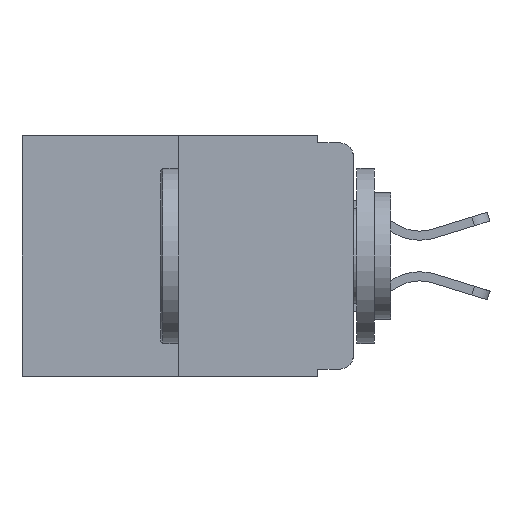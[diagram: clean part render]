
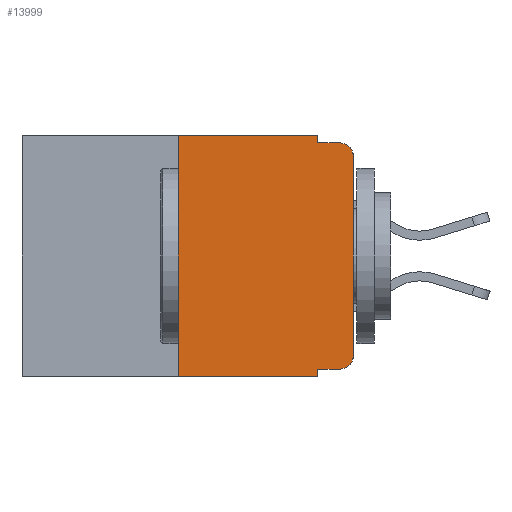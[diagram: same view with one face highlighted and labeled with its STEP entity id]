
A CAD part, left-side view. The second image highlights one B-rep face of the part: STEP entity #13999.
In plain terms, the highlighted planar face has unit normal (-1, 0, 0).
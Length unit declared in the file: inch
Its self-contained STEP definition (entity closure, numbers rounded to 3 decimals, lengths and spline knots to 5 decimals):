
#170 = CARTESIAN_POINT ( 'NONE',  ( 0., 0., -0.313 ) ) ;
#595 = EDGE_CURVE ( 'NONE', #14541, #14249, #4104, .T. ) ;
#627 = DIRECTION ( 'NONE',  ( 0., 0., -1. ) ) ;
#764 = VERTEX_POINT ( 'NONE', #4735 ) ;
#1036 = CARTESIAN_POINT ( 'NONE',  ( 0., 0.051, -0.343 ) ) ;
#1538 = CARTESIAN_POINT ( 'NONE',  ( 0., 0.051, -0.333 ) ) ;
#2058 = CARTESIAN_POINT ( 'NONE',  ( 0., 0.25, 0. ) ) ;
#2104 = CARTESIAN_POINT ( 'NONE',  ( 0., 0.051, 0. ) ) ;
#2351 = VECTOR ( 'NONE', #6844, 39.37008 ) ;
#2370 = VECTOR ( 'NONE', #8442, 39.37008 ) ;
#2421 = EDGE_CURVE ( 'NONE', #15066, #16653, #8781, .T. ) ;
#2644 = VECTOR ( 'NONE', #10840, 39.37008 ) ;
#3401 = CARTESIAN_POINT ( 'NONE',  ( 0., 0.051, 0. ) ) ;
#3480 = CARTESIAN_POINT ( 'NONE',  ( 0., 0.02, -0.313 ) ) ;
#3957 = AXIS2_PLACEMENT_3D ( 'NONE', #16062, #11904, #13245 ) ;
#4104 = CIRCLE ( 'NONE', #15993, 0.02 ) ;
#4123 = DIRECTION ( 'NONE',  ( 0., -1., 0. ) ) ;
#4286 = ORIENTED_EDGE ( 'NONE', *, *, #595, .T. ) ;
#4735 = CARTESIAN_POINT ( 'NONE',  ( 0., 0., -0.03 ) ) ;
#4946 = EDGE_CURVE ( 'NONE', #12644, #6397, #11073, .T. ) ;
#5188 = CARTESIAN_POINT ( 'NONE',  ( 0., 0.25, 0. ) ) ;
#5298 = ORIENTED_EDGE ( 'NONE', *, *, #17246, .F. ) ;
#5504 = CARTESIAN_POINT ( 'NONE',  ( 0., 0.051, 0. ) ) ;
#5694 = LINE ( 'NONE', #1538, #16495 ) ;
#5914 = FACE_OUTER_BOUND ( 'NONE', #6399, .T. ) ;
#6042 = ORIENTED_EDGE ( 'NONE', *, *, #4946, .F. ) ;
#6061 = DIRECTION ( 'NONE',  ( 0., -1., 0. ) ) ;
#6142 = CARTESIAN_POINT ( 'NONE',  ( 0., 0.02, -0.333 ) ) ;
#6217 = LINE ( 'NONE', #8803, #7564 ) ;
#6397 = VERTEX_POINT ( 'NONE', #13373 ) ;
#6399 = EDGE_LOOP ( 'NONE', ( #8392, #15746, #17805, #6042, #5298, #8787, #16891, #14525, #8882, #4286 ) ) ;
#6556 = EDGE_CURVE ( 'NONE', #7332, #14581, #12127, .T. ) ;
#6844 = DIRECTION ( 'NONE',  ( 0., 0., 1. ) ) ;
#6945 = CIRCLE ( 'NONE', #9717, 0.02 ) ;
#7332 = VERTEX_POINT ( 'NONE', #9834 ) ;
#7340 = LINE ( 'NONE', #10999, #2370 ) ;
#7564 = VECTOR ( 'NONE', #6061, 39.37008 ) ;
#7791 = VERTEX_POINT ( 'NONE', #17828 ) ;
#8173 = CARTESIAN_POINT ( 'NONE',  ( 0., 0.051, -0.01 ) ) ;
#8340 = DIRECTION ( 'NONE',  ( 0., -1., 0. ) ) ;
#8392 = ORIENTED_EDGE ( 'NONE', *, *, #17815, .T. ) ;
#8442 = DIRECTION ( 'NONE',  ( 0., -1., 0. ) ) ;
#8781 = LINE ( 'NONE', #5504, #13330 ) ;
#8787 = ORIENTED_EDGE ( 'NONE', *, *, #6556, .F. ) ;
#8803 = CARTESIAN_POINT ( 'NONE',  ( 0., 0.473, -0.343 ) ) ;
#8882 = ORIENTED_EDGE ( 'NONE', *, *, #14210, .T. ) ;
#9075 = VECTOR ( 'NONE', #8340, 39.37008 ) ;
#9501 = DIRECTION ( 'NONE',  ( 0., 0., -1. ) ) ;
#9717 = AXIS2_PLACEMENT_3D ( 'NONE', #17316, #16001, #14624 ) ;
#9834 = CARTESIAN_POINT ( 'NONE',  ( 0., 0.25, -0.343 ) ) ;
#10254 = DIRECTION ( 'NONE',  ( 0., 0., -1. ) ) ;
#10840 = DIRECTION ( 'NONE',  ( 0., 0., 1. ) ) ;
#10854 = CARTESIAN_POINT ( 'NONE',  ( 0., 0., 0. ) ) ;
#10999 = CARTESIAN_POINT ( 'NONE',  ( 0., 0.473, 0. ) ) ;
#11073 = LINE ( 'NONE', #3401, #13444 ) ;
#11733 = PLANE ( 'NONE',  #3957 ) ;
#11904 = DIRECTION ( 'NONE',  ( 1., 0., 0. ) ) ;
#12127 = LINE ( 'NONE', #5188, #2644 ) ;
#12268 = EDGE_CURVE ( 'NONE', #764, #7791, #6945, .T. ) ;
#12644 = VERTEX_POINT ( 'NONE', #2104 ) ;
#12970 = CARTESIAN_POINT ( 'NONE',  ( 0., 0.051, -0.333 ) ) ;
#13245 = DIRECTION ( 'NONE',  ( 0., 0., -1. ) ) ;
#13330 = VECTOR ( 'NONE', #9501, 39.37008 ) ;
#13373 = CARTESIAN_POINT ( 'NONE',  ( 0., 0.051, -0.01 ) ) ;
#13376 = LINE ( 'NONE', #10854, #2351 ) ;
#13444 = VECTOR ( 'NONE', #627, 39.37008 ) ;
#13999 = ADVANCED_FACE ( 'NONE', ( #5914 ), #11733, .F. ) ;
#14210 = EDGE_CURVE ( 'NONE', #15066, #14541, #5694, .T. ) ;
#14249 = VERTEX_POINT ( 'NONE', #170 ) ;
#14361 = DIRECTION ( 'NONE',  ( -1., 0., 0. ) ) ;
#14525 = ORIENTED_EDGE ( 'NONE', *, *, #2421, .F. ) ;
#14541 = VERTEX_POINT ( 'NONE', #6142 ) ;
#14581 = VERTEX_POINT ( 'NONE', #2058 ) ;
#14624 = DIRECTION ( 'NONE',  ( 0., 0., -1. ) ) ;
#15066 = VERTEX_POINT ( 'NONE', #12970 ) ;
#15746 = ORIENTED_EDGE ( 'NONE', *, *, #12268, .T. ) ;
#15993 = AXIS2_PLACEMENT_3D ( 'NONE', #3480, #14361, #10254 ) ;
#16001 = DIRECTION ( 'NONE',  ( -1., 0., 0. ) ) ;
#16062 = CARTESIAN_POINT ( 'NONE',  ( 0., 0.473, 0. ) ) ;
#16121 = EDGE_CURVE ( 'NONE', #6397, #7791, #16425, .T. ) ;
#16425 = LINE ( 'NONE', #8173, #9075 ) ;
#16495 = VECTOR ( 'NONE', #4123, 39.37008 ) ;
#16653 = VERTEX_POINT ( 'NONE', #1036 ) ;
#16891 = ORIENTED_EDGE ( 'NONE', *, *, #16961, .T. ) ;
#16961 = EDGE_CURVE ( 'NONE', #7332, #16653, #6217, .T. ) ;
#17246 = EDGE_CURVE ( 'NONE', #14581, #12644, #7340, .T. ) ;
#17316 = CARTESIAN_POINT ( 'NONE',  ( 0., 0.02, -0.03 ) ) ;
#17805 = ORIENTED_EDGE ( 'NONE', *, *, #16121, .F. ) ;
#17815 = EDGE_CURVE ( 'NONE', #14249, #764, #13376, .T. ) ;
#17828 = CARTESIAN_POINT ( 'NONE',  ( 0., 0.02, -0.01 ) ) ;
